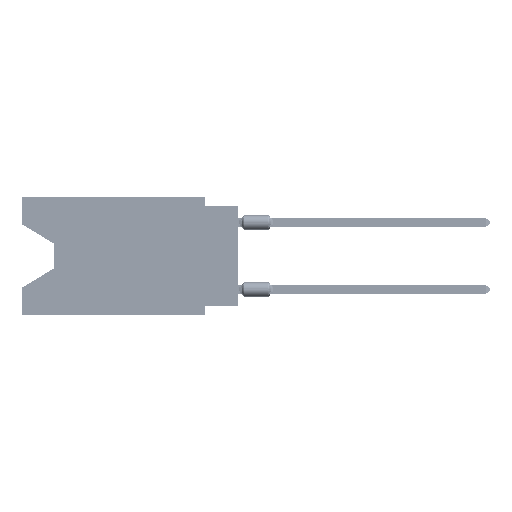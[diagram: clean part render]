
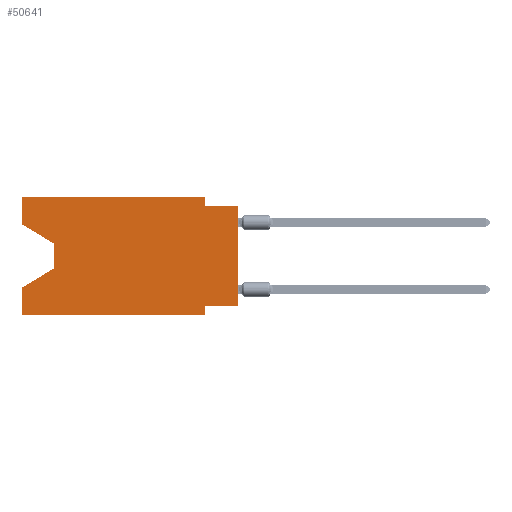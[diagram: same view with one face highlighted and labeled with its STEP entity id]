
A CAD part, left-side view. The second image highlights one B-rep face of the part: STEP entity #50641.
In plain terms, the highlighted planar face has unit normal (-1, 0, 0).
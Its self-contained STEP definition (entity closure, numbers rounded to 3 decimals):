
#1080 = DIRECTION ( 'NONE',  ( 1., 0., 0. ) ) ;
#1674 = VECTOR ( 'NONE', #12955, 1000. ) ;
#1850 = CARTESIAN_POINT ( 'NONE',  ( 0., 2.54, -8.89 ) ) ;
#1965 = LINE ( 'NONE', #69422, #63939 ) ;
#2280 = LINE ( 'NONE', #61846, #47249 ) ;
#2919 = VERTEX_POINT ( 'NONE', #40472 ) ;
#3460 = CARTESIAN_POINT ( 'NONE',  ( 0., 2.54, 0. ) ) ;
#5494 = VERTEX_POINT ( 'NONE', #59190 ) ;
#5890 = LINE ( 'NONE', #6661, #9427 ) ;
#6661 = CARTESIAN_POINT ( 'NONE',  ( 0., 16.383, 0. ) ) ;
#6699 = VECTOR ( 'NONE', #29144, 1000. ) ;
#7200 = VERTEX_POINT ( 'NONE', #53642 ) ;
#7254 = LINE ( 'NONE', #54880, #59705 ) ;
#7432 = VERTEX_POINT ( 'NONE', #3460 ) ;
#7776 = DIRECTION ( 'NONE',  ( 0., 0., -1. ) ) ;
#9427 = VECTOR ( 'NONE', #48346, 1000. ) ;
#9820 = DIRECTION ( 'NONE',  ( 0., -1., 0. ) ) ;
#11578 = ORIENTED_EDGE ( 'NONE', *, *, #29468, .T. ) ;
#12955 = DIRECTION ( 'NONE',  ( 0., -1., 0. ) ) ;
#13737 = LINE ( 'NONE', #26429, #16222 ) ;
#13767 = CARTESIAN_POINT ( 'NONE',  ( 0., 16.383, 0. ) ) ;
#16222 = VECTOR ( 'NONE', #7776, 1000. ) ;
#16449 = VERTEX_POINT ( 'NONE', #36687 ) ;
#18333 = VECTOR ( 'NONE', #56646, 1000. ) ;
#19120 = ORIENTED_EDGE ( 'NONE', *, *, #45763, .F. ) ;
#19415 = EDGE_CURVE ( 'NONE', #2919, #76411, #2280, .T. ) ;
#20568 = CARTESIAN_POINT ( 'NONE',  ( 0., 16.383, -8.89 ) ) ;
#21162 = EDGE_CURVE ( 'NONE', #46715, #76411, #7254, .T. ) ;
#22158 = ORIENTED_EDGE ( 'NONE', *, *, #73914, .T. ) ;
#22664 = LINE ( 'NONE', #57608, #59205 ) ;
#22755 = CARTESIAN_POINT ( 'NONE',  ( 0., 2.54, -8.255 ) ) ;
#22791 = LINE ( 'NONE', #35487, #6699 ) ;
#23039 = EDGE_CURVE ( 'NONE', #31255, #16449, #22791, .T. ) ;
#24873 = CARTESIAN_POINT ( 'NONE',  ( 0., 16.383, 0. ) ) ;
#25698 = CARTESIAN_POINT ( 'NONE',  ( 0., 13.97, -5.385 ) ) ;
#26180 = DIRECTION ( 'NONE',  ( 0., 1., 0. ) ) ;
#26429 = CARTESIAN_POINT ( 'NONE',  ( 0., 2.54, -8.89 ) ) ;
#26458 = PLANE ( 'NONE',  #77032 ) ;
#29144 = DIRECTION ( 'NONE',  ( 0., -0.855, -0.519 ) ) ;
#29329 = CARTESIAN_POINT ( 'NONE',  ( 0., 16.383, -2.038 ) ) ;
#29468 = EDGE_CURVE ( 'NONE', #16449, #62806, #22664, .T. ) ;
#30992 = DIRECTION ( 'NONE',  ( 0., 0., -1. ) ) ;
#31255 = VERTEX_POINT ( 'NONE', #29329 ) ;
#33044 = VERTEX_POINT ( 'NONE', #22755 ) ;
#33159 = ORIENTED_EDGE ( 'NONE', *, *, #42212, .F. ) ;
#35487 = CARTESIAN_POINT ( 'NONE',  ( 0., 16.383, -2.038 ) ) ;
#36687 = CARTESIAN_POINT ( 'NONE',  ( 0., 13.97, -3.505 ) ) ;
#36945 = LINE ( 'NONE', #44473, #49930 ) ;
#37697 = VERTEX_POINT ( 'NONE', #1850 ) ;
#37863 = EDGE_CURVE ( 'NONE', #31255, #73573, #40333, .T. ) ;
#38156 = CARTESIAN_POINT ( 'NONE',  ( 0., 0., -0.635 ) ) ;
#38460 = ORIENTED_EDGE ( 'NONE', *, *, #63932, .F. ) ;
#40333 = LINE ( 'NONE', #40715, #75964 ) ;
#40472 = CARTESIAN_POINT ( 'NONE',  ( 0., 0., -8.255 ) ) ;
#40573 = EDGE_CURVE ( 'NONE', #62806, #7200, #55862, .T. ) ;
#40715 = CARTESIAN_POINT ( 'NONE',  ( 0., 16.383, 0. ) ) ;
#41149 = CARTESIAN_POINT ( 'NONE',  ( 0., 13.97, -5.385 ) ) ;
#41840 = ORIENTED_EDGE ( 'NONE', *, *, #40573, .T. ) ;
#42212 = EDGE_CURVE ( 'NONE', #5494, #7200, #5890, .T. ) ;
#42559 = VECTOR ( 'NONE', #9820, 1000. ) ;
#43955 = FACE_OUTER_BOUND ( 'NONE', #52302, .T. ) ;
#44473 = CARTESIAN_POINT ( 'NONE',  ( 0., 2.54, 0. ) ) ;
#44714 = DIRECTION ( 'NONE',  ( 0., 0., -1. ) ) ;
#45763 = EDGE_CURVE ( 'NONE', #73573, #7432, #49866, .T. ) ;
#46715 = VERTEX_POINT ( 'NONE', #60809 ) ;
#47249 = VECTOR ( 'NONE', #50713, 1000. ) ;
#48155 = ORIENTED_EDGE ( 'NONE', *, *, #55523, .F. ) ;
#48346 = DIRECTION ( 'NONE',  ( 0., 0., 1. ) ) ;
#49866 = LINE ( 'NONE', #24873, #1674 ) ;
#49930 = VECTOR ( 'NONE', #30992, 1000. ) ;
#50641 = ADVANCED_FACE ( 'NONE', ( #43955 ), #26458, .F. ) ;
#50713 = DIRECTION ( 'NONE',  ( 0., 0., 1. ) ) ;
#50736 = LINE ( 'NONE', #20568, #42559 ) ;
#51216 = CARTESIAN_POINT ( 'NONE',  ( 0., 16.383, 0. ) ) ;
#52010 = EDGE_CURVE ( 'NONE', #2919, #33044, #1965, .T. ) ;
#52302 = EDGE_LOOP ( 'NONE', ( #75255, #11578, #41840, #33159, #22158, #48155, #68102, #63531, #60084, #38460, #19120, #59738 ) ) ;
#53642 = CARTESIAN_POINT ( 'NONE',  ( 0., 16.383, -6.852 ) ) ;
#54490 = DIRECTION ( 'NONE',  ( 0., -1., 0. ) ) ;
#54880 = CARTESIAN_POINT ( 'NONE',  ( 0., 0., -0.635 ) ) ;
#55523 = EDGE_CURVE ( 'NONE', #33044, #37697, #13737, .T. ) ;
#55862 = LINE ( 'NONE', #25698, #18333 ) ;
#56646 = DIRECTION ( 'NONE',  ( 0., 0.855, -0.519 ) ) ;
#57608 = CARTESIAN_POINT ( 'NONE',  ( 0., 13.97, -3.505 ) ) ;
#58384 = DIRECTION ( 'NONE',  ( 0., 0., -1. ) ) ;
#59190 = CARTESIAN_POINT ( 'NONE',  ( 0., 16.383, -8.89 ) ) ;
#59205 = VECTOR ( 'NONE', #58384, 1000. ) ;
#59705 = VECTOR ( 'NONE', #54490, 1000. ) ;
#59738 = ORIENTED_EDGE ( 'NONE', *, *, #37863, .F. ) ;
#60084 = ORIENTED_EDGE ( 'NONE', *, *, #21162, .F. ) ;
#60809 = CARTESIAN_POINT ( 'NONE',  ( 0., 2.54, -0.635 ) ) ;
#61846 = CARTESIAN_POINT ( 'NONE',  ( 0., 0., 0. ) ) ;
#62806 = VERTEX_POINT ( 'NONE', #41149 ) ;
#63531 = ORIENTED_EDGE ( 'NONE', *, *, #19415, .T. ) ;
#63932 = EDGE_CURVE ( 'NONE', #7432, #46715, #36945, .T. ) ;
#63939 = VECTOR ( 'NONE', #26180, 1000. ) ;
#64906 = DIRECTION ( 'NONE',  ( 0., 0., 1. ) ) ;
#68102 = ORIENTED_EDGE ( 'NONE', *, *, #52010, .F. ) ;
#69422 = CARTESIAN_POINT ( 'NONE',  ( 0., 0., -8.255 ) ) ;
#73573 = VERTEX_POINT ( 'NONE', #51216 ) ;
#73914 = EDGE_CURVE ( 'NONE', #5494, #37697, #50736, .T. ) ;
#75255 = ORIENTED_EDGE ( 'NONE', *, *, #23039, .T. ) ;
#75964 = VECTOR ( 'NONE', #64906, 1000. ) ;
#76411 = VERTEX_POINT ( 'NONE', #38156 ) ;
#77032 = AXIS2_PLACEMENT_3D ( 'NONE', #13767, #1080, #44714 ) ;
